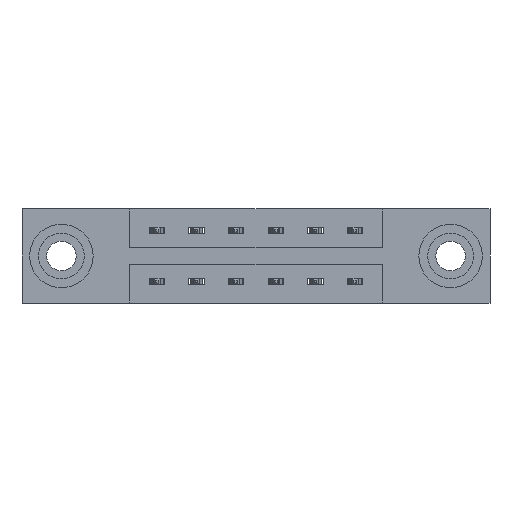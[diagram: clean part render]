
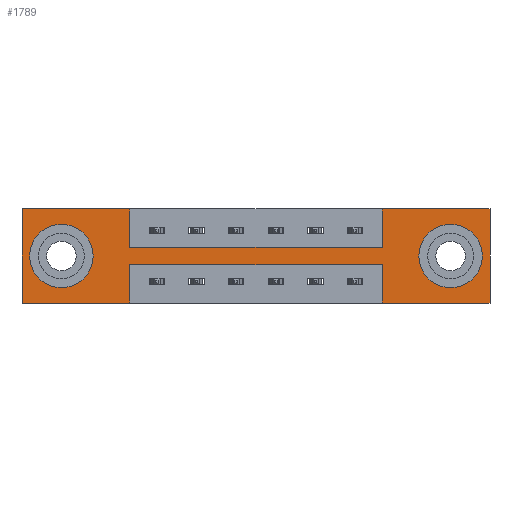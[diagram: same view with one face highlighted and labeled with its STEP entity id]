
A CAD part, front view. The second image highlights one B-rep face of the part: STEP entity #1789.
In plain terms, the highlighted planar face has unit normal (0, -1, 0).
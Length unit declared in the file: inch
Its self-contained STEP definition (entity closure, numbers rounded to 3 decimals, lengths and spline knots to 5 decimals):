
#93 = CARTESIAN_POINT ( 'NONE',  ( 0.425, 0., 0. ) ) ;
#137 = LINE ( 'NONE', #8621, #4589 ) ;
#170 = DIRECTION ( 'NONE',  ( 0., 0., 1. ) ) ;
#203 = CARTESIAN_POINT ( 'NONE',  ( 0., 0., 0. ) ) ;
#215 = VERTEX_POINT ( 'NONE', #8088 ) ;
#220 = VERTEX_POINT ( 'NONE', #7968 ) ;
#230 = VERTEX_POINT ( 'NONE', #8844 ) ;
#284 = EDGE_CURVE ( 'NONE', #4505, #230, #6657, .T. ) ;
#306 = VECTOR ( 'NONE', #2648, 39.37008 ) ;
#334 = CARTESIAN_POINT ( 'NONE',  ( 0.425, 0., -0.37 ) ) ;
#385 = DIRECTION ( 'NONE',  ( 1., 0., 0. ) ) ;
#505 = VERTEX_POINT ( 'NONE', #6667 ) ;
#547 = VECTOR ( 'NONE', #4825, 39.37008 ) ;
#557 = ORIENTED_EDGE ( 'NONE', *, *, #4938, .T. ) ;
#598 = VERTEX_POINT ( 'NONE', #9210 ) ;
#662 = VERTEX_POINT ( 'NONE', #334 ) ;
#730 = FACE_OUTER_BOUND ( 'NONE', #8254, .T. ) ;
#766 = VECTOR ( 'NONE', #7420, 39.37008 ) ;
#842 = CARTESIAN_POINT ( 'NONE',  ( 1.417, 0., -0.37 ) ) ;
#861 = ORIENTED_EDGE ( 'NONE', *, *, #8033, .F. ) ;
#1058 = LINE ( 'NONE', #5906, #766 ) ;
#1141 = ORIENTED_EDGE ( 'NONE', *, *, #284, .F. ) ;
#1181 = EDGE_LOOP ( 'NONE', ( #8818, #557 ) ) ;
#1269 = AXIS2_PLACEMENT_3D ( 'NONE', #4263, #9316, #5088 ) ;
#1360 = AXIS2_PLACEMENT_3D ( 'NONE', #4519, #5753, #3797 ) ;
#1416 = ORIENTED_EDGE ( 'NONE', *, *, #5321, .F. ) ;
#1487 = VERTEX_POINT ( 'NONE', #5689 ) ;
#1568 = VERTEX_POINT ( 'NONE', #2077 ) ;
#1720 = DIRECTION ( 'NONE',  ( 0., 1., 0. ) ) ;
#1789 = ADVANCED_FACE ( 'NONE', ( #7136, #5119, #730 ), #4541, .T. ) ;
#2077 = CARTESIAN_POINT ( 'NONE',  ( 0.425, 0., -0.22 ) ) ;
#2084 = CARTESIAN_POINT ( 'NONE',  ( 1.842, 0., 0. ) ) ;
#2142 = VERTEX_POINT ( 'NONE', #8980 ) ;
#2648 = DIRECTION ( 'NONE',  ( 0., 0., 1. ) ) ;
#2733 = LINE ( 'NONE', #842, #306 ) ;
#2748 = EDGE_CURVE ( 'NONE', #2142, #9261, #8014, .T. ) ;
#2851 = DIRECTION ( 'NONE',  ( 0., 0., -1. ) ) ;
#2972 = ORIENTED_EDGE ( 'NONE', *, *, #6967, .F. ) ;
#3128 = CARTESIAN_POINT ( 'NONE',  ( 1.417, 0., -0.15 ) ) ;
#3270 = DIRECTION ( 'NONE',  ( 1., 0., 0. ) ) ;
#3272 = LINE ( 'NONE', #8436, #547 ) ;
#3311 = CARTESIAN_POINT ( 'NONE',  ( 0., 0., -0.37 ) ) ;
#3454 = VECTOR ( 'NONE', #8117, 39.37008 ) ;
#3548 = VECTOR ( 'NONE', #2851, 39.37008 ) ;
#3738 = CARTESIAN_POINT ( 'NONE',  ( 1.687, 0., -0.185 ) ) ;
#3797 = DIRECTION ( 'NONE',  ( 0., 0., -1. ) ) ;
#3940 = VECTOR ( 'NONE', #385, 39.37008 ) ;
#3969 = AXIS2_PLACEMENT_3D ( 'NONE', #9556, #5413, #170 ) ;
#4184 = DIRECTION ( 'NONE',  ( 0., 0., 1. ) ) ;
#4263 = CARTESIAN_POINT ( 'NONE',  ( 0.155, 0., -0.185 ) ) ;
#4366 = VECTOR ( 'NONE', #4997, 39.37008 ) ;
#4496 = CARTESIAN_POINT ( 'NONE',  ( 0., 0., 0. ) ) ;
#4505 = VERTEX_POINT ( 'NONE', #93 ) ;
#4519 = CARTESIAN_POINT ( 'NONE',  ( 0., 0., -0.37 ) ) ;
#4541 = PLANE ( 'NONE',  #1360 ) ;
#4579 = DIRECTION ( 'NONE',  ( 0., 0., -1. ) ) ;
#4589 = VECTOR ( 'NONE', #4184, 39.37008 ) ;
#4671 = CARTESIAN_POINT ( 'NONE',  ( 0., 0., 0. ) ) ;
#4808 = EDGE_CURVE ( 'NONE', #9922, #1487, #6686, .T. ) ;
#4825 = DIRECTION ( 'NONE',  ( 0., 0., -1. ) ) ;
#4896 = VECTOR ( 'NONE', #7066, 39.37008 ) ;
#4938 = EDGE_CURVE ( 'NONE', #6534, #598, #6567, .T. ) ;
#4985 = ORIENTED_EDGE ( 'NONE', *, *, #6411, .T. ) ;
#4997 = DIRECTION ( 'NONE',  ( -1., 0., 0. ) ) ;
#5088 = DIRECTION ( 'NONE',  ( 0., 0., 1. ) ) ;
#5119 = FACE_BOUND ( 'NONE', #1181, .T. ) ;
#5228 = ORIENTED_EDGE ( 'NONE', *, *, #5307, .F. ) ;
#5304 = DIRECTION ( 'NONE',  ( 0., 0., 1. ) ) ;
#5307 = EDGE_CURVE ( 'NONE', #215, #1568, #5868, .T. ) ;
#5321 = EDGE_CURVE ( 'NONE', #662, #7374, #1058, .T. ) ;
#5334 = LINE ( 'NONE', #4496, #8702 ) ;
#5413 = DIRECTION ( 'NONE',  ( 0., 1., 0. ) ) ;
#5455 = ORIENTED_EDGE ( 'NONE', *, *, #2748, .F. ) ;
#5469 = DIRECTION ( 'NONE',  ( 1., 0., 0. ) ) ;
#5689 = CARTESIAN_POINT ( 'NONE',  ( 1.687, 0., -0.107 ) ) ;
#5705 = CARTESIAN_POINT ( 'NONE',  ( 0.425, 0., -0.15 ) ) ;
#5753 = DIRECTION ( 'NONE',  ( 0., -1., 0. ) ) ;
#5838 = CIRCLE ( 'NONE', #1269, 0.078 ) ;
#5868 = LINE ( 'NONE', #7389, #3454 ) ;
#5906 = CARTESIAN_POINT ( 'NONE',  ( 0., 0., -0.37 ) ) ;
#5936 = EDGE_CURVE ( 'NONE', #505, #9371, #9940, .T. ) ;
#6283 = EDGE_CURVE ( 'NONE', #9371, #215, #2733, .T. ) ;
#6394 = VECTOR ( 'NONE', #5469, 39.37008 ) ;
#6411 = EDGE_CURVE ( 'NONE', #1487, #9922, #7568, .T. ) ;
#6531 = VECTOR ( 'NONE', #3270, 39.37008 ) ;
#6534 = VERTEX_POINT ( 'NONE', #8469 ) ;
#6567 = CIRCLE ( 'NONE', #3969, 0.078 ) ;
#6657 = LINE ( 'NONE', #7089, #4896 ) ;
#6667 = CARTESIAN_POINT ( 'NONE',  ( 1.842, 0., -0.37 ) ) ;
#6672 = EDGE_CURVE ( 'NONE', #230, #7142, #8415, .T. ) ;
#6681 = CARTESIAN_POINT ( 'NONE',  ( 1.687, 0., -0.185 ) ) ;
#6686 = CIRCLE ( 'NONE', #9844, 0.078 ) ;
#6748 = EDGE_CURVE ( 'NONE', #598, #6534, #5838, .T. ) ;
#6812 = EDGE_LOOP ( 'NONE', ( #4985, #6995 ) ) ;
#6967 = EDGE_CURVE ( 'NONE', #1568, #662, #9391, .T. ) ;
#6995 = ORIENTED_EDGE ( 'NONE', *, *, #4808, .T. ) ;
#7066 = DIRECTION ( 'NONE',  ( 0., 0., -1. ) ) ;
#7070 = CARTESIAN_POINT ( 'NONE',  ( 1.417, 0., -0.37 ) ) ;
#7089 = CARTESIAN_POINT ( 'NONE',  ( 0.425, 0., 0. ) ) ;
#7136 = FACE_BOUND ( 'NONE', #6812, .T. ) ;
#7142 = VERTEX_POINT ( 'NONE', #3128 ) ;
#7167 = CARTESIAN_POINT ( 'NONE',  ( 0., 0., -0.37 ) ) ;
#7235 = ORIENTED_EDGE ( 'NONE', *, *, #6283, .F. ) ;
#7374 = VERTEX_POINT ( 'NONE', #7167 ) ;
#7389 = CARTESIAN_POINT ( 'NONE',  ( 0.425, 0., -0.22 ) ) ;
#7420 = DIRECTION ( 'NONE',  ( -1., 0., 0. ) ) ;
#7430 = DIRECTION ( 'NONE',  ( 0., 0., -1. ) ) ;
#7435 = ORIENTED_EDGE ( 'NONE', *, *, #7546, .F. ) ;
#7546 = EDGE_CURVE ( 'NONE', #7142, #2142, #137, .T. ) ;
#7568 = CIRCLE ( 'NONE', #8165, 0.078 ) ;
#7583 = CARTESIAN_POINT ( 'NONE',  ( 0.425, 0., -0.37 ) ) ;
#7650 = ORIENTED_EDGE ( 'NONE', *, *, #7960, .F. ) ;
#7960 = EDGE_CURVE ( 'NONE', #220, #4505, #9912, .T. ) ;
#7968 = CARTESIAN_POINT ( 'NONE',  ( 0., 0., 0. ) ) ;
#8014 = LINE ( 'NONE', #203, #3940 ) ;
#8033 = EDGE_CURVE ( 'NONE', #9261, #505, #3272, .T. ) ;
#8088 = CARTESIAN_POINT ( 'NONE',  ( 1.417, 0., -0.22 ) ) ;
#8117 = DIRECTION ( 'NONE',  ( -1., 0., 0. ) ) ;
#8165 = AXIS2_PLACEMENT_3D ( 'NONE', #3738, #8935, #4579 ) ;
#8254 = EDGE_LOOP ( 'NONE', ( #2972, #5228, #7235, #9004, #861, #5455, #7435, #9208, #1141, #7650, #9381, #1416 ) ) ;
#8415 = LINE ( 'NONE', #5705, #6531 ) ;
#8424 = EDGE_CURVE ( 'NONE', #7374, #220, #5334, .T. ) ;
#8436 = CARTESIAN_POINT ( 'NONE',  ( 1.842, 0., 0. ) ) ;
#8469 = CARTESIAN_POINT ( 'NONE',  ( 0.155, 0., -0.263 ) ) ;
#8621 = CARTESIAN_POINT ( 'NONE',  ( 1.417, 0., 0. ) ) ;
#8702 = VECTOR ( 'NONE', #5304, 39.37008 ) ;
#8818 = ORIENTED_EDGE ( 'NONE', *, *, #6748, .T. ) ;
#8844 = CARTESIAN_POINT ( 'NONE',  ( 0.425, 0., -0.15 ) ) ;
#8935 = DIRECTION ( 'NONE',  ( 0., 1., 0. ) ) ;
#8980 = CARTESIAN_POINT ( 'NONE',  ( 1.417, 0., 0. ) ) ;
#9004 = ORIENTED_EDGE ( 'NONE', *, *, #5936, .F. ) ;
#9208 = ORIENTED_EDGE ( 'NONE', *, *, #6672, .F. ) ;
#9210 = CARTESIAN_POINT ( 'NONE',  ( 0.155, 0., -0.107 ) ) ;
#9261 = VERTEX_POINT ( 'NONE', #2084 ) ;
#9316 = DIRECTION ( 'NONE',  ( 0., 1., 0. ) ) ;
#9371 = VERTEX_POINT ( 'NONE', #7070 ) ;
#9381 = ORIENTED_EDGE ( 'NONE', *, *, #8424, .F. ) ;
#9391 = LINE ( 'NONE', #7583, #3548 ) ;
#9556 = CARTESIAN_POINT ( 'NONE',  ( 0.155, 0., -0.185 ) ) ;
#9844 = AXIS2_PLACEMENT_3D ( 'NONE', #6681, #1720, #7430 ) ;
#9895 = CARTESIAN_POINT ( 'NONE',  ( 1.687, 0., -0.263 ) ) ;
#9912 = LINE ( 'NONE', #4671, #6394 ) ;
#9922 = VERTEX_POINT ( 'NONE', #9895 ) ;
#9940 = LINE ( 'NONE', #3311, #4366 ) ;
